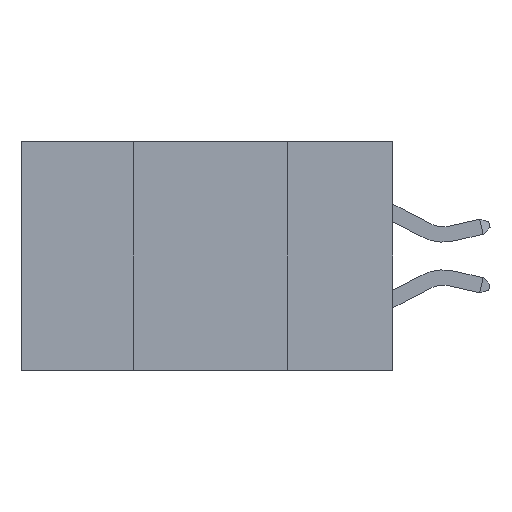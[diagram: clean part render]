
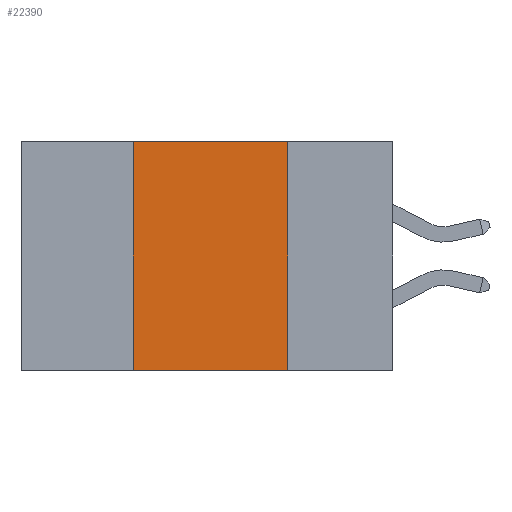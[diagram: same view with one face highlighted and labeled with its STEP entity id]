
A CAD part, left-side view. The second image highlights one B-rep face of the part: STEP entity #22390.
In plain terms, the highlighted planar face has unit normal (-1, 0, 0).
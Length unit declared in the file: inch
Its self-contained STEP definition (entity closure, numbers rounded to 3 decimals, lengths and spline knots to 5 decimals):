
#1284 = DIRECTION ( 'NONE',  ( 0., 0., 1. ) ) ;
#1803 = VERTEX_POINT ( 'NONE', #9591 ) ;
#2973 = CARTESIAN_POINT ( 'NONE',  ( 0., 0.6, 0. ) ) ;
#3403 = DIRECTION ( 'NONE',  ( 0., -1., 0. ) ) ;
#3716 = VECTOR ( 'NONE', #3403, 39.37008 ) ;
#5412 = CARTESIAN_POINT ( 'NONE',  ( 0., 0.6, -0.37 ) ) ;
#6928 = ORIENTED_EDGE ( 'NONE', *, *, #7498, .F. ) ;
#7498 = EDGE_CURVE ( 'NONE', #17032, #12911, #17039, .T. ) ;
#7738 = AXIS2_PLACEMENT_3D ( 'NONE', #2973, #10514, #8734 ) ;
#8551 = LINE ( 'NONE', #15741, #12406 ) ;
#8734 = DIRECTION ( 'NONE',  ( 0., 0., -1. ) ) ;
#9591 = CARTESIAN_POINT ( 'NONE',  ( 0., 0.17, -0.37 ) ) ;
#9704 = ORIENTED_EDGE ( 'NONE', *, *, #11132, .T. ) ;
#10265 = CARTESIAN_POINT ( 'NONE',  ( 0., 0.17, 0. ) ) ;
#10514 = DIRECTION ( 'NONE',  ( 1., 0., 0. ) ) ;
#11132 = EDGE_CURVE ( 'NONE', #12008, #1803, #12854, .T. ) ;
#11653 = CARTESIAN_POINT ( 'NONE',  ( 0., 0.42, 0. ) ) ;
#11925 = EDGE_CURVE ( 'NONE', #12911, #1803, #8551, .T. ) ;
#12008 = VERTEX_POINT ( 'NONE', #18004 ) ;
#12406 = VECTOR ( 'NONE', #22975, 39.37008 ) ;
#12854 = LINE ( 'NONE', #5412, #3716 ) ;
#12911 = VERTEX_POINT ( 'NONE', #10265 ) ;
#13277 = EDGE_LOOP ( 'NONE', ( #19323, #6928, #19527, #9704 ) ) ;
#14281 = PLANE ( 'NONE',  #7738 ) ;
#14465 = VECTOR ( 'NONE', #1284, 39.37008 ) ;
#15741 = CARTESIAN_POINT ( 'NONE',  ( 0., 0.17, 0. ) ) ;
#17032 = VERTEX_POINT ( 'NONE', #11653 ) ;
#17039 = LINE ( 'NONE', #22956, #20594 ) ;
#17729 = FACE_OUTER_BOUND ( 'NONE', #13277, .T. ) ;
#18004 = CARTESIAN_POINT ( 'NONE',  ( 0., 0.42, -0.37 ) ) ;
#18396 = EDGE_CURVE ( 'NONE', #12008, #17032, #22679, .T. ) ;
#18952 = DIRECTION ( 'NONE',  ( 0., -1., 0. ) ) ;
#19323 = ORIENTED_EDGE ( 'NONE', *, *, #11925, .F. ) ;
#19527 = ORIENTED_EDGE ( 'NONE', *, *, #18396, .F. ) ;
#20594 = VECTOR ( 'NONE', #18952, 39.37008 ) ;
#22390 = ADVANCED_FACE ( 'NONE', ( #17729 ), #14281, .F. ) ;
#22679 = LINE ( 'NONE', #22794, #14465 ) ;
#22794 = CARTESIAN_POINT ( 'NONE',  ( 0., 0.42, 0. ) ) ;
#22956 = CARTESIAN_POINT ( 'NONE',  ( 0., 0.6, 0. ) ) ;
#22975 = DIRECTION ( 'NONE',  ( 0., 0., -1. ) ) ;
